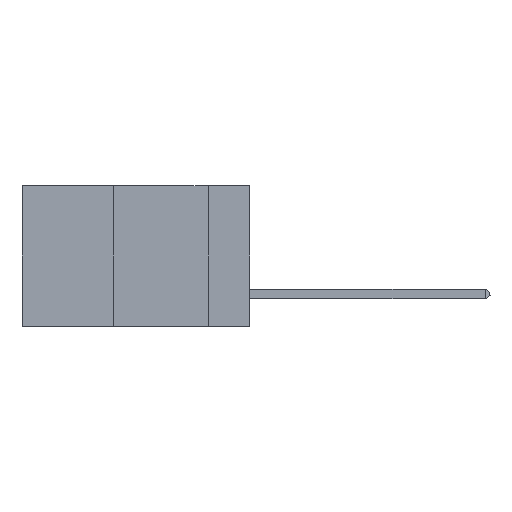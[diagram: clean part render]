
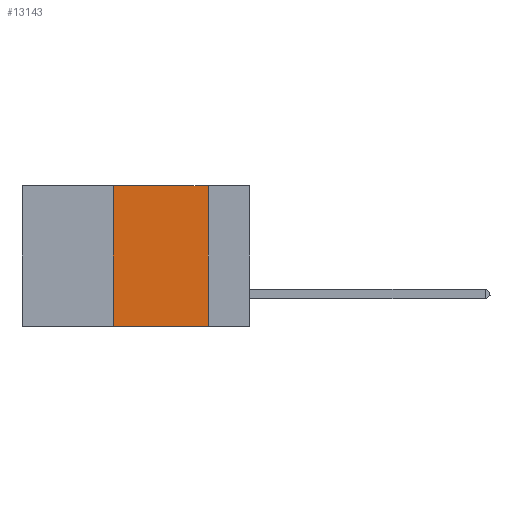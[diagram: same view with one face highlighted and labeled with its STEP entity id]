
A CAD part, left-side view. The second image highlights one B-rep face of the part: STEP entity #13143.
In plain terms, the highlighted planar face has unit normal (-1, 0, 0).
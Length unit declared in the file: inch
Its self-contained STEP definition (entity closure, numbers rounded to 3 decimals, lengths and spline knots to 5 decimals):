
#302 = LINE ( 'NONE', #9590, #23943 ) ;
#1572 = VECTOR ( 'NONE', #21785, 39.37008 ) ;
#1636 = DIRECTION ( 'NONE',  ( 0., 0., -1. ) ) ;
#4282 = ORIENTED_EDGE ( 'NONE', *, *, #22608, .F. ) ;
#5261 = LINE ( 'NONE', #19400, #1572 ) ;
#5973 = LINE ( 'NONE', #11119, #29933 ) ;
#7102 = VERTEX_POINT ( 'NONE', #16458 ) ;
#7297 = CARTESIAN_POINT ( 'NONE',  ( 0., 0.11, -0.37 ) ) ;
#8188 = DIRECTION ( 'NONE',  ( 0., -1., 0. ) ) ;
#8369 = PLANE ( 'NONE',  #16993 ) ;
#8903 = EDGE_LOOP ( 'NONE', ( #4282, #15760, #11891, #10301 ) ) ;
#9590 = CARTESIAN_POINT ( 'NONE',  ( 0., 0.6, -0.37 ) ) ;
#10301 = ORIENTED_EDGE ( 'NONE', *, *, #28270, .T. ) ;
#11119 = CARTESIAN_POINT ( 'NONE',  ( 0., 0.11, 0. ) ) ;
#11752 = DIRECTION ( 'NONE',  ( 0., -1., 0. ) ) ;
#11891 = ORIENTED_EDGE ( 'NONE', *, *, #25461, .F. ) ;
#12312 = EDGE_CURVE ( 'NONE', #16517, #7102, #29314, .T. ) ;
#12990 = CARTESIAN_POINT ( 'NONE',  ( 0., 0.36, -0.37 ) ) ;
#13143 = ADVANCED_FACE ( 'NONE', ( #26018 ), #8369, .F. ) ;
#15760 = ORIENTED_EDGE ( 'NONE', *, *, #12312, .F. ) ;
#16458 = CARTESIAN_POINT ( 'NONE',  ( 0., 0.11, 0. ) ) ;
#16517 = VERTEX_POINT ( 'NONE', #25188 ) ;
#16993 = AXIS2_PLACEMENT_3D ( 'NONE', #29870, #18311, #1636 ) ;
#17624 = CARTESIAN_POINT ( 'NONE',  ( 0., 0.6, 0. ) ) ;
#18311 = DIRECTION ( 'NONE',  ( 1., 0., 0. ) ) ;
#19400 = CARTESIAN_POINT ( 'NONE',  ( 0., 0.36, 0. ) ) ;
#19701 = VERTEX_POINT ( 'NONE', #12990 ) ;
#20181 = VECTOR ( 'NONE', #8188, 39.37008 ) ;
#20521 = DIRECTION ( 'NONE',  ( 0., 0., -1. ) ) ;
#21785 = DIRECTION ( 'NONE',  ( 0., 0., 1. ) ) ;
#22608 = EDGE_CURVE ( 'NONE', #7102, #26803, #5973, .T. ) ;
#23943 = VECTOR ( 'NONE', #11752, 39.37008 ) ;
#25188 = CARTESIAN_POINT ( 'NONE',  ( 0., 0.36, 0. ) ) ;
#25461 = EDGE_CURVE ( 'NONE', #19701, #16517, #5261, .T. ) ;
#26018 = FACE_OUTER_BOUND ( 'NONE', #8903, .T. ) ;
#26803 = VERTEX_POINT ( 'NONE', #7297 ) ;
#28270 = EDGE_CURVE ( 'NONE', #19701, #26803, #302, .T. ) ;
#29314 = LINE ( 'NONE', #17624, #20181 ) ;
#29870 = CARTESIAN_POINT ( 'NONE',  ( 0., 0.6, 0. ) ) ;
#29933 = VECTOR ( 'NONE', #20521, 39.37008 ) ;
